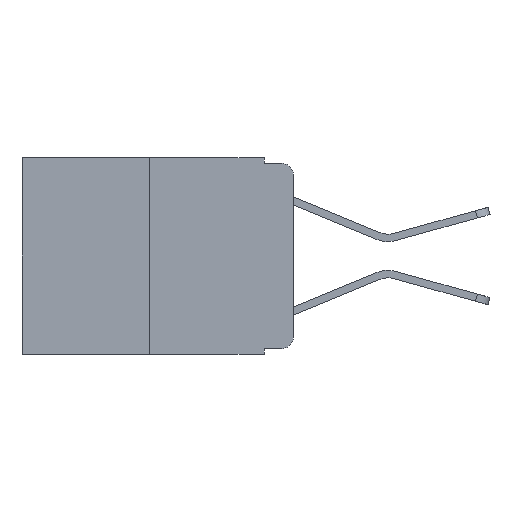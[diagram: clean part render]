
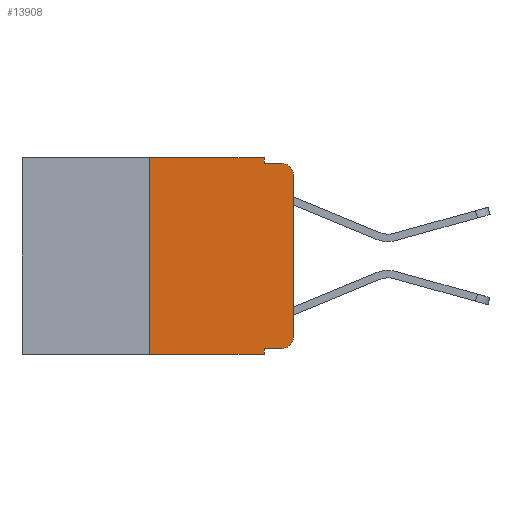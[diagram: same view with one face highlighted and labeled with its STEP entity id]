
A CAD part, left-side view. The second image highlights one B-rep face of the part: STEP entity #13908.
In plain terms, the highlighted planar face has unit normal (-1, 0, 0).
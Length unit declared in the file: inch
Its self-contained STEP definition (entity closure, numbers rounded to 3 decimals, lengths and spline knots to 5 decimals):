
#163 = VERTEX_POINT ( 'NONE', #9064 ) ;
#1043 = ORIENTED_EDGE ( 'NONE', *, *, #18571, .T. ) ;
#1116 = CARTESIAN_POINT ( 'NONE',  ( 0., 0.25, 0. ) ) ;
#1345 = EDGE_CURVE ( 'NONE', #21745, #17819, #19631, .T. ) ;
#1707 = VERTEX_POINT ( 'NONE', #2543 ) ;
#2410 = CARTESIAN_POINT ( 'NONE',  ( 0., 0.051, 0. ) ) ;
#2436 = ORIENTED_EDGE ( 'NONE', *, *, #9194, .T. ) ;
#2543 = CARTESIAN_POINT ( 'NONE',  ( 0., 0., -0.313 ) ) ;
#2712 = CARTESIAN_POINT ( 'NONE',  ( 0., 0., 0. ) ) ;
#2731 = DIRECTION ( 'NONE',  ( 0., -1., 0. ) ) ;
#3124 = DIRECTION ( 'NONE',  ( 0., 0., 1. ) ) ;
#3437 = LINE ( 'NONE', #7302, #17996 ) ;
#3491 = DIRECTION ( 'NONE',  ( 0., -1., 0. ) ) ;
#3560 = VECTOR ( 'NONE', #16298, 39.37008 ) ;
#4097 = LINE ( 'NONE', #11039, #11483 ) ;
#4568 = CARTESIAN_POINT ( 'NONE',  ( 0., 0.473, 0. ) ) ;
#4663 = VERTEX_POINT ( 'NONE', #21180 ) ;
#5215 = VECTOR ( 'NONE', #3124, 39.37008 ) ;
#5384 = ORIENTED_EDGE ( 'NONE', *, *, #9736, .T. ) ;
#5706 = ORIENTED_EDGE ( 'NONE', *, *, #17825, .F. ) ;
#6432 = DIRECTION ( 'NONE',  ( -1., 0., 0. ) ) ;
#6574 = DIRECTION ( 'NONE',  ( 1., 0., 0. ) ) ;
#7119 = DIRECTION ( 'NONE',  ( 0., 0., -1. ) ) ;
#7302 = CARTESIAN_POINT ( 'NONE',  ( 0., 0.051, -0.01 ) ) ;
#7379 = CARTESIAN_POINT ( 'NONE',  ( 0., 0.02, -0.01 ) ) ;
#7927 = CARTESIAN_POINT ( 'NONE',  ( 0., 0.051, -0.343 ) ) ;
#8942 = VECTOR ( 'NONE', #2731, 39.37008 ) ;
#9064 = CARTESIAN_POINT ( 'NONE',  ( 0., 0.051, -0.01 ) ) ;
#9194 = EDGE_CURVE ( 'NONE', #11078, #16462, #19779, .T. ) ;
#9262 = CARTESIAN_POINT ( 'NONE',  ( 0., 0.02, -0.333 ) ) ;
#9736 = EDGE_CURVE ( 'NONE', #19015, #14635, #10772, .T. ) ;
#10220 = LINE ( 'NONE', #2410, #11119 ) ;
#10246 = ORIENTED_EDGE ( 'NONE', *, *, #12676, .T. ) ;
#10772 = LINE ( 'NONE', #12395, #8942 ) ;
#11039 = CARTESIAN_POINT ( 'NONE',  ( 0., 0.051, 0. ) ) ;
#11078 = VERTEX_POINT ( 'NONE', #21158 ) ;
#11119 = VECTOR ( 'NONE', #24107, 39.37008 ) ;
#11483 = VECTOR ( 'NONE', #7119, 39.37008 ) ;
#12395 = CARTESIAN_POINT ( 'NONE',  ( 0., 0.051, -0.333 ) ) ;
#12484 = PLANE ( 'NONE',  #13818 ) ;
#12676 = EDGE_CURVE ( 'NONE', #1707, #11078, #16541, .T. ) ;
#12808 = CARTESIAN_POINT ( 'NONE',  ( 0., 0.25, -0.343 ) ) ;
#13818 = AXIS2_PLACEMENT_3D ( 'NONE', #4568, #6574, #24345 ) ;
#13869 = LINE ( 'NONE', #1116, #5215 ) ;
#13908 = ADVANCED_FACE ( 'NONE', ( #21356 ), #12484, .F. ) ;
#13951 = ORIENTED_EDGE ( 'NONE', *, *, #20506, .F. ) ;
#14635 = VERTEX_POINT ( 'NONE', #9262 ) ;
#14692 = DIRECTION ( 'NONE',  ( -1., 0., 0. ) ) ;
#15378 = AXIS2_PLACEMENT_3D ( 'NONE', #16935, #14692, #24868 ) ;
#15924 = VECTOR ( 'NONE', #16656, 39.37008 ) ;
#16298 = DIRECTION ( 'NONE',  ( 0., 0., 1. ) ) ;
#16462 = VERTEX_POINT ( 'NONE', #7379 ) ;
#16541 = LINE ( 'NONE', #2712, #3560 ) ;
#16656 = DIRECTION ( 'NONE',  ( 0., -1., 0. ) ) ;
#16935 = CARTESIAN_POINT ( 'NONE',  ( 0., 0.02, -0.03 ) ) ;
#17179 = ORIENTED_EDGE ( 'NONE', *, *, #1345, .T. ) ;
#17472 = ORIENTED_EDGE ( 'NONE', *, *, #22177, .F. ) ;
#17819 = VERTEX_POINT ( 'NONE', #7927 ) ;
#17825 = EDGE_CURVE ( 'NONE', #23959, #4663, #19593, .T. ) ;
#17996 = VECTOR ( 'NONE', #3491, 39.37008 ) ;
#18508 = AXIS2_PLACEMENT_3D ( 'NONE', #24365, #6432, #22223 ) ;
#18571 = EDGE_CURVE ( 'NONE', #14635, #1707, #25105, .T. ) ;
#19015 = VERTEX_POINT ( 'NONE', #23408 ) ;
#19053 = ORIENTED_EDGE ( 'NONE', *, *, #19670, .F. ) ;
#19573 = DIRECTION ( 'NONE',  ( 0., -1., 0. ) ) ;
#19593 = LINE ( 'NONE', #23732, #20223 ) ;
#19631 = LINE ( 'NONE', #22540, #15924 ) ;
#19670 = EDGE_CURVE ( 'NONE', #163, #16462, #3437, .T. ) ;
#19779 = CIRCLE ( 'NONE', #15378, 0.02 ) ;
#20223 = VECTOR ( 'NONE', #19573, 39.37008 ) ;
#20506 = EDGE_CURVE ( 'NONE', #4663, #163, #4097, .T. ) ;
#21158 = CARTESIAN_POINT ( 'NONE',  ( 0., 0., -0.03 ) ) ;
#21180 = CARTESIAN_POINT ( 'NONE',  ( 0., 0.051, 0. ) ) ;
#21356 = FACE_OUTER_BOUND ( 'NONE', #22408, .T. ) ;
#21745 = VERTEX_POINT ( 'NONE', #12808 ) ;
#22177 = EDGE_CURVE ( 'NONE', #19015, #17819, #10220, .T. ) ;
#22223 = DIRECTION ( 'NONE',  ( 0., 0., -1. ) ) ;
#22408 = EDGE_LOOP ( 'NONE', ( #10246, #2436, #19053, #13951, #5706, #22660, #17179, #17472, #5384, #1043 ) ) ;
#22540 = CARTESIAN_POINT ( 'NONE',  ( 0., 0.473, -0.343 ) ) ;
#22660 = ORIENTED_EDGE ( 'NONE', *, *, #24423, .F. ) ;
#23408 = CARTESIAN_POINT ( 'NONE',  ( 0., 0.051, -0.333 ) ) ;
#23732 = CARTESIAN_POINT ( 'NONE',  ( 0., 0.473, 0. ) ) ;
#23959 = VERTEX_POINT ( 'NONE', #24922 ) ;
#24107 = DIRECTION ( 'NONE',  ( 0., 0., -1. ) ) ;
#24345 = DIRECTION ( 'NONE',  ( 0., 0., -1. ) ) ;
#24365 = CARTESIAN_POINT ( 'NONE',  ( 0., 0.02, -0.313 ) ) ;
#24423 = EDGE_CURVE ( 'NONE', #21745, #23959, #13869, .T. ) ;
#24868 = DIRECTION ( 'NONE',  ( 0., 0., -1. ) ) ;
#24922 = CARTESIAN_POINT ( 'NONE',  ( 0., 0.25, 0. ) ) ;
#25105 = CIRCLE ( 'NONE', #18508, 0.02 ) ;
